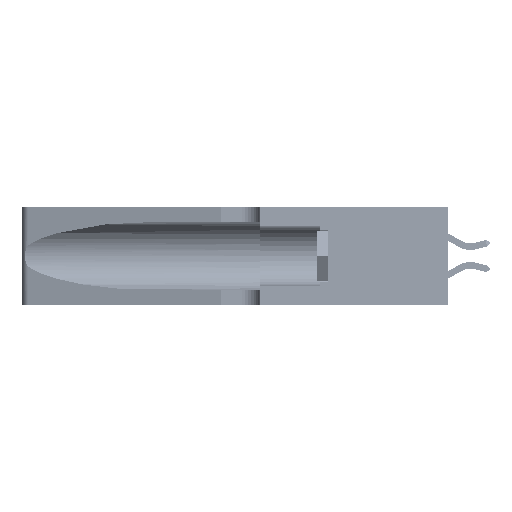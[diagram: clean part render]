
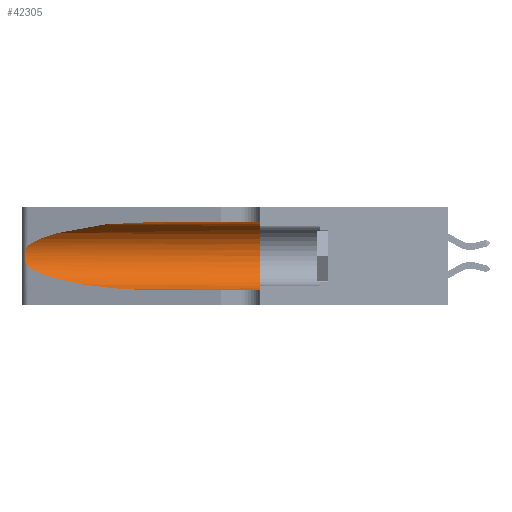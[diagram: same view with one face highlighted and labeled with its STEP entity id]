
A CAD part, left-side view. The second image highlights one B-rep face of the part: STEP entity #42305.
In plain terms, the highlighted cylindrical face has radius 3.308 mm (diameter 6.617 mm), a partial arc.
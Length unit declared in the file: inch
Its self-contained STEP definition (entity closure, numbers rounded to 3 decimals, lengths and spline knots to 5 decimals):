
#129 = EDGE_CURVE ( 'NONE', #36935, #7854, #26347, .T. ) ;
#576 = CARTESIAN_POINT ( 'NONE',  ( 0.2373, 1.15595, 0.08982 ) ) ;
#917 = CARTESIAN_POINT ( 'NONE',  ( 0.25487, 1.22718, 0.14631 ) ) ;
#939 = AXIS2_PLACEMENT_3D ( 'NONE', #5397, #40560, #24896 ) ;
#1546 = CARTESIAN_POINT ( 'NONE',  ( 0.26075, 1.23896, 0.19203 ) ) ;
#3165 = DIRECTION ( 'NONE',  ( 0., -1., 0. ) ) ;
#4441 = CARTESIAN_POINT ( 'NONE',  ( 0.1305, 0.72297, 0.05475 ) ) ;
#5397 = CARTESIAN_POINT ( 'NONE',  ( 0.1305, 1.61858, 0.185 ) ) ;
#5432 = CARTESIAN_POINT ( 'NONE',  ( 0.25487, 1.22718, 0.14631 ) ) ;
#5641 = VERTEX_POINT ( 'NONE', #20148 ) ;
#5764 = CARTESIAN_POINT ( 'NONE',  ( 0.26017, 1.23833, 0.17102 ) ) ;
#6786 = LINE ( 'NONE', #17329, #17661 ) ;
#7854 = VERTEX_POINT ( 'NONE', #12994 ) ;
#8894 = CARTESIAN_POINT ( 'NONE',  ( 0.1305, 0.35, 0.185 ) ) ;
#9279 = CARTESIAN_POINT ( 'NONE',  ( 0.25639, 1.23184, 0.21858 ) ) ;
#9475 = EDGE_CURVE ( 'NONE', #7854, #39222, #33399, .T. ) ;
#10686 = EDGE_LOOP ( 'NONE', ( #11564, #40106, #31655, #35172, #16809, #44236 ) ) ;
#11111 = AXIS2_PLACEMENT_3D ( 'NONE', #8894, #16492, #20046 ) ;
#11183 = CARTESIAN_POINT ( 'NONE',  ( 0.18966, 0.96281, 0.31525 ) ) ;
#11564 = ORIENTED_EDGE ( 'NONE', *, *, #15116, .T. ) ;
#12994 = CARTESIAN_POINT ( 'NONE',  ( 0.1305, 0.35, 0.31525 ) ) ;
#13653 = CARTESIAN_POINT ( 'NONE',  ( 0.25856, 1.23593, 0.16098 ) ) ;
#14121 = VERTEX_POINT ( 'NONE', #24058 ) ;
#15116 = EDGE_CURVE ( 'NONE', #36935, #5641, #33536, .T. ) ;
#16492 = DIRECTION ( 'NONE',  ( 0., 1., 0. ) ) ;
#16809 = ORIENTED_EDGE ( 'NONE', *, *, #9475, .F. ) ;
#17196 = CARTESIAN_POINT ( 'NONE',  ( 0.25854, 1.2359, 0.20912 ) ) ;
#17329 = CARTESIAN_POINT ( 'NONE',  ( 0.1305, 1.61858, 0.05475 ) ) ;
#17357 = CARTESIAN_POINT ( 'NONE',  ( 0.25555, 1.22993, 0.14849 ) ) ;
#17661 = VECTOR ( 'NONE', #3165, 39.37008 ) ;
#20046 = DIRECTION ( 'NONE',  ( 0., 0., 1. ) ) ;
#20148 = CARTESIAN_POINT ( 'NONE',  ( 0.25487, 1.22718, 0.22369 ) ) ;
#21146 = B_SPLINE_CURVE_WITH_KNOTS ( 'NONE', 3,
 ( #24589, #40424, #9279, #28968, #17196, #28635, #1546, #29141, #5764, #13653, #40592, #28467, #17357, #5432 ),
 .UNSPECIFIED., .F., .F.,
 ( 4, 2, 2, 2, 2, 2, 4 ),
 ( 0., 0.00027, 0.00053, 0.00107, 0.0016, 0.00187, 0.00214 ),
 .UNSPECIFIED. ) ;
#21189 = VERTEX_POINT ( 'NONE', #32129 ) ;
#22155 = CARTESIAN_POINT ( 'NONE',  ( 0.1305, 0.72297, 0.31525 ) ) ;
#24058 = CARTESIAN_POINT ( 'NONE',  ( 0.25487, 1.22718, 0.14631 ) ) ;
#24589 = CARTESIAN_POINT ( 'NONE',  ( 0.25487, 1.22718, 0.22369 ) ) ;
#24896 = DIRECTION ( 'NONE',  ( 0., 0., -1. ) ) ;
#26347 = LINE ( 'NONE', #28226, #39597 ) ;
#28007 = CARTESIAN_POINT ( 'NONE',  ( 0.18966, 0.96281, 0.05475 ) ) ;
#28226 = CARTESIAN_POINT ( 'NONE',  ( 0.1305, 1.61858, 0.31525 ) ) ;
#28386 = DIRECTION ( 'NONE',  ( 0., -1., 0. ) ) ;
#28467 = CARTESIAN_POINT ( 'NONE',  ( 0.25639, 1.23186, 0.15144 ) ) ;
#28635 = CARTESIAN_POINT ( 'NONE',  ( 0.26018, 1.23835, 0.19895 ) ) ;
#28680 = CARTESIAN_POINT ( 'NONE',  ( 0.1305, 0.35, 0.05475 ) ) ;
#28968 = CARTESIAN_POINT ( 'NONE',  ( 0.25787, 1.23484, 0.2124 ) ) ;
#29141 = CARTESIAN_POINT ( 'NONE',  ( 0.26075, 1.23896, 0.178 ) ) ;
#30084 = FACE_OUTER_BOUND ( 'NONE', #10686, .T. ) ;
#30915 = EDGE_CURVE ( 'NONE', #21189, #39222, #6786, .T. ) ;
#31029 =( BOUNDED_CURVE ( )  B_SPLINE_CURVE ( 3, ( #917, #576, #28007, #4441 ),
 .UNSPECIFIED., .F., .T. ) 
 B_SPLINE_CURVE_WITH_KNOTS ( ( 4, 4 ),
 ( 3.44316, 4.71239 ),
 .UNSPECIFIED. ) 
 CURVE ( )  GEOMETRIC_REPRESENTATION_ITEM ( )  RATIONAL_B_SPLINE_CURVE ( ( 1., 0.87, 0.87, 1. ) ) 
 REPRESENTATION_ITEM ( '' )  );
#31655 = ORIENTED_EDGE ( 'NONE', *, *, #41385, .T. ) ;
#32129 = CARTESIAN_POINT ( 'NONE',  ( 0.1305, 0.72297, 0.05475 ) ) ;
#33399 = CIRCLE ( 'NONE', #11111, 0.13025 ) ;
#33536 =( BOUNDED_CURVE ( )  B_SPLINE_CURVE ( 3, ( #33753, #11183, #37654, #37977 ),
 .UNSPECIFIED., .F., .F. ) 
 B_SPLINE_CURVE_WITH_KNOTS ( ( 4, 4 ),
 ( 1.5708, 2.84003 ),
 .UNSPECIFIED. ) 
 CURVE ( )  GEOMETRIC_REPRESENTATION_ITEM ( )  RATIONAL_B_SPLINE_CURVE ( ( 1., 0.87, 0.87, 1. ) ) 
 REPRESENTATION_ITEM ( '' )  );
#33753 = CARTESIAN_POINT ( 'NONE',  ( 0.1305, 0.72297, 0.31525 ) ) ;
#35172 = ORIENTED_EDGE ( 'NONE', *, *, #30915, .T. ) ;
#36935 = VERTEX_POINT ( 'NONE', #22155 ) ;
#37654 = CARTESIAN_POINT ( 'NONE',  ( 0.2373, 1.15595, 0.28018 ) ) ;
#37977 = CARTESIAN_POINT ( 'NONE',  ( 0.25487, 1.22718, 0.22369 ) ) ;
#39222 = VERTEX_POINT ( 'NONE', #28680 ) ;
#39597 = VECTOR ( 'NONE', #28386, 39.37008 ) ;
#40106 = ORIENTED_EDGE ( 'NONE', *, *, #49259, .T. ) ;
#40424 = CARTESIAN_POINT ( 'NONE',  ( 0.25555, 1.22994, 0.2215 ) ) ;
#40560 = DIRECTION ( 'NONE',  ( 0., -1., 0. ) ) ;
#40592 = CARTESIAN_POINT ( 'NONE',  ( 0.25789, 1.23486, 0.15765 ) ) ;
#41385 = EDGE_CURVE ( 'NONE', #14121, #21189, #31029, .T. ) ;
#42145 = CYLINDRICAL_SURFACE ( 'NONE', #939, 0.13025 ) ;
#42305 = ADVANCED_FACE ( 'NONE', ( #30084 ), #42145, .F. ) ;
#44236 = ORIENTED_EDGE ( 'NONE', *, *, #129, .F. ) ;
#49259 = EDGE_CURVE ( 'NONE', #5641, #14121, #21146, .T. ) ;
